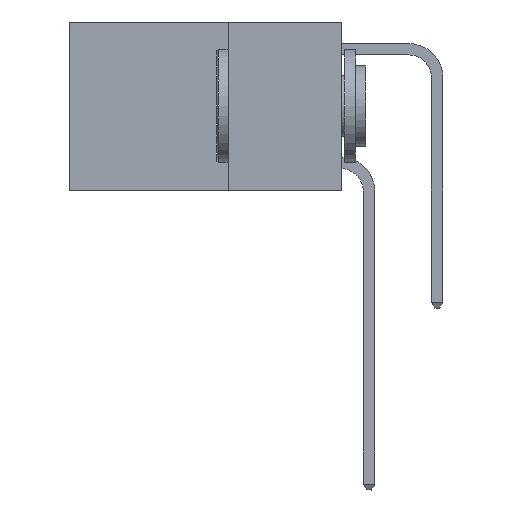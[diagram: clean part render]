
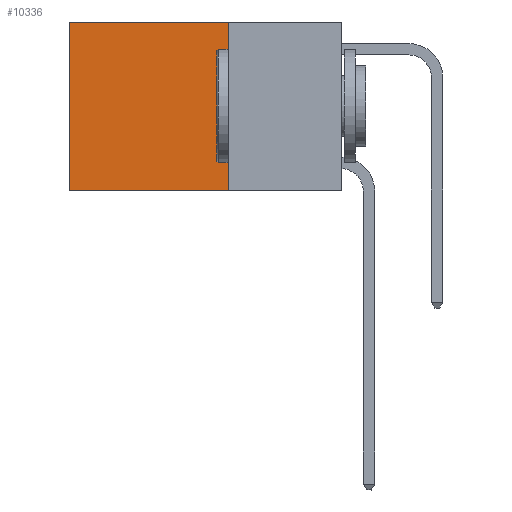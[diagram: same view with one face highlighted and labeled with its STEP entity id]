
A CAD part, left-side view. The second image highlights one B-rep face of the part: STEP entity #10336.
In plain terms, the highlighted planar face has unit normal (-1, 0, 0).
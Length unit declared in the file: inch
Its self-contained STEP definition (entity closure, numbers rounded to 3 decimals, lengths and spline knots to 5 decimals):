
#326 = CARTESIAN_POINT ( 'NONE',  ( 0.2625, 0.6, -0.37 ) ) ;
#576 = VECTOR ( 'NONE', #24249, 39.37008 ) ;
#5694 = DIRECTION ( 'NONE',  ( 1., 0., 0. ) ) ;
#8057 = VERTEX_POINT ( 'NONE', #12617 ) ;
#9310 = EDGE_LOOP ( 'NONE', ( #15480, #26043, #10771, #10507 ) ) ;
#9861 = LINE ( 'NONE', #18589, #28153 ) ;
#10336 = ADVANCED_FACE ( 'NONE', ( #19010 ), #20847, .F. ) ;
#10507 = ORIENTED_EDGE ( 'NONE', *, *, #22116, .T. ) ;
#10763 = CARTESIAN_POINT ( 'NONE',  ( 0.2625, 0.25, 0. ) ) ;
#10771 = ORIENTED_EDGE ( 'NONE', *, *, #23896, .F. ) ;
#10966 = CARTESIAN_POINT ( 'NONE',  ( 0.2625, 0.25, 0. ) ) ;
#11980 = CARTESIAN_POINT ( 'NONE',  ( 0.2625, 0.25, 0. ) ) ;
#12617 = CARTESIAN_POINT ( 'NONE',  ( 0.2625, 0.6, 0. ) ) ;
#13419 = VECTOR ( 'NONE', #24366, 39.37008 ) ;
#13702 = VERTEX_POINT ( 'NONE', #10763 ) ;
#13815 = EDGE_CURVE ( 'NONE', #17135, #19446, #9861, .T. ) ;
#15431 = CARTESIAN_POINT ( 'NONE',  ( 0.2625, 0.25, -0.37 ) ) ;
#15480 = ORIENTED_EDGE ( 'NONE', *, *, #25679, .T. ) ;
#17135 = VERTEX_POINT ( 'NONE', #15431 ) ;
#18589 = CARTESIAN_POINT ( 'NONE',  ( 0.2625, 0.25, -0.37 ) ) ;
#19010 = FACE_OUTER_BOUND ( 'NONE', #9310, .T. ) ;
#19446 = VERTEX_POINT ( 'NONE', #326 ) ;
#20208 = VECTOR ( 'NONE', #24703, 39.37008 ) ;
#20847 = PLANE ( 'NONE',  #26775 ) ;
#21274 = DIRECTION ( 'NONE',  ( 0., 0., -1. ) ) ;
#22116 = EDGE_CURVE ( 'NONE', #13702, #8057, #26844, .T. ) ;
#22697 = CARTESIAN_POINT ( 'NONE',  ( 0.2625, 0.25, 0. ) ) ;
#22870 = DIRECTION ( 'NONE',  ( 0., 1., 0. ) ) ;
#23896 = EDGE_CURVE ( 'NONE', #13702, #17135, #26403, .T. ) ;
#24226 = CARTESIAN_POINT ( 'NONE',  ( 0.2625, 0.6, 0. ) ) ;
#24249 = DIRECTION ( 'NONE',  ( 0., 0., -1. ) ) ;
#24366 = DIRECTION ( 'NONE',  ( 0., 0., -1. ) ) ;
#24703 = DIRECTION ( 'NONE',  ( 0., 1., 0. ) ) ;
#25679 = EDGE_CURVE ( 'NONE', #8057, #19446, #26791, .T. ) ;
#26043 = ORIENTED_EDGE ( 'NONE', *, *, #13815, .F. ) ;
#26403 = LINE ( 'NONE', #10966, #576 ) ;
#26775 = AXIS2_PLACEMENT_3D ( 'NONE', #11980, #5694, #21274 ) ;
#26791 = LINE ( 'NONE', #24226, #13419 ) ;
#26844 = LINE ( 'NONE', #22697, #20208 ) ;
#28153 = VECTOR ( 'NONE', #22870, 39.37008 ) ;
